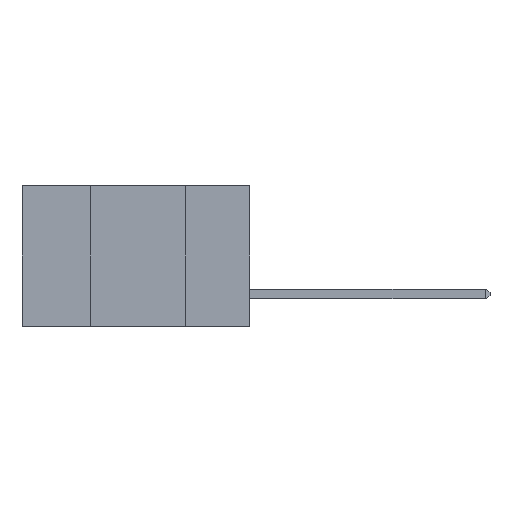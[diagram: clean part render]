
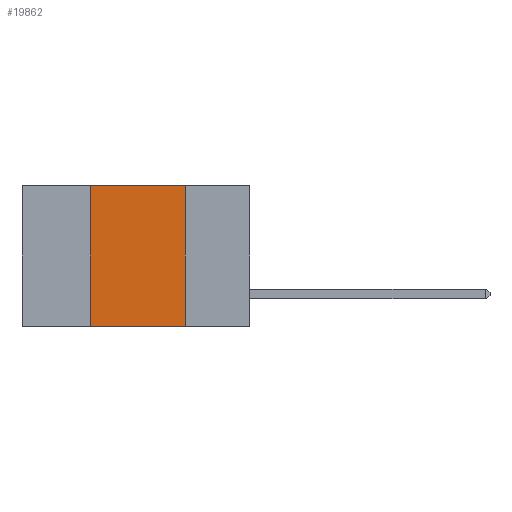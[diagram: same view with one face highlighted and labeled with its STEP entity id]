
A CAD part, left-side view. The second image highlights one B-rep face of the part: STEP entity #19862.
In plain terms, the highlighted planar face has unit normal (-1, 0, 0).
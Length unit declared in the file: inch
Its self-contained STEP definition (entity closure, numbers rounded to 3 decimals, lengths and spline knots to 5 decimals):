
#846 = DIRECTION ( 'NONE',  ( 0., 0., -1. ) ) ;
#2176 = EDGE_CURVE ( 'NONE', #30953, #27593, #3510, .T. ) ;
#3510 = LINE ( 'NONE', #15400, #28170 ) ;
#3720 = DIRECTION ( 'NONE',  ( 1., 0., 0. ) ) ;
#4038 = LINE ( 'NONE', #5726, #22422 ) ;
#5726 = CARTESIAN_POINT ( 'NONE',  ( 0., 0.6, -0.37 ) ) ;
#5980 = EDGE_CURVE ( 'NONE', #27593, #22082, #21764, .T. ) ;
#7221 = CARTESIAN_POINT ( 'NONE',  ( 0., 0.42, -0.37 ) ) ;
#7526 = VERTEX_POINT ( 'NONE', #7221 ) ;
#9014 = EDGE_CURVE ( 'NONE', #7526, #22082, #4038, .T. ) ;
#11180 = FACE_OUTER_BOUND ( 'NONE', #17814, .T. ) ;
#11453 = VECTOR ( 'NONE', #13572, 39.37008 ) ;
#13572 = DIRECTION ( 'NONE',  ( 0., 0., 1. ) ) ;
#14864 = DIRECTION ( 'NONE',  ( 0., -1., 0. ) ) ;
#15057 = EDGE_CURVE ( 'NONE', #7526, #30953, #17039, .T. ) ;
#15400 = CARTESIAN_POINT ( 'NONE',  ( 0., 0.6, 0. ) ) ;
#15410 = DIRECTION ( 'NONE',  ( 0., -1., 0. ) ) ;
#15531 = CARTESIAN_POINT ( 'NONE',  ( 0., 0.17, 0. ) ) ;
#17039 = LINE ( 'NONE', #18266, #11453 ) ;
#17814 = EDGE_LOOP ( 'NONE', ( #21784, #23199, #23093, #25374 ) ) ;
#18196 = CARTESIAN_POINT ( 'NONE',  ( 0., 0.6, 0. ) ) ;
#18266 = CARTESIAN_POINT ( 'NONE',  ( 0., 0.42, 0. ) ) ;
#19267 = CARTESIAN_POINT ( 'NONE',  ( 0., 0.17, -0.37 ) ) ;
#19862 = ADVANCED_FACE ( 'NONE', ( #11180 ), #27534, .F. ) ;
#20590 = DIRECTION ( 'NONE',  ( 0., 0., -1. ) ) ;
#21764 = LINE ( 'NONE', #22627, #27974 ) ;
#21784 = ORIENTED_EDGE ( 'NONE', *, *, #5980, .F. ) ;
#21849 = AXIS2_PLACEMENT_3D ( 'NONE', #18196, #3720, #20590 ) ;
#22082 = VERTEX_POINT ( 'NONE', #19267 ) ;
#22314 = CARTESIAN_POINT ( 'NONE',  ( 0., 0.42, 0. ) ) ;
#22422 = VECTOR ( 'NONE', #15410, 39.37008 ) ;
#22627 = CARTESIAN_POINT ( 'NONE',  ( 0., 0.17, 0. ) ) ;
#23093 = ORIENTED_EDGE ( 'NONE', *, *, #15057, .F. ) ;
#23199 = ORIENTED_EDGE ( 'NONE', *, *, #2176, .F. ) ;
#25374 = ORIENTED_EDGE ( 'NONE', *, *, #9014, .T. ) ;
#27534 = PLANE ( 'NONE',  #21849 ) ;
#27593 = VERTEX_POINT ( 'NONE', #15531 ) ;
#27974 = VECTOR ( 'NONE', #846, 39.37008 ) ;
#28170 = VECTOR ( 'NONE', #14864, 39.37008 ) ;
#30953 = VERTEX_POINT ( 'NONE', #22314 ) ;
